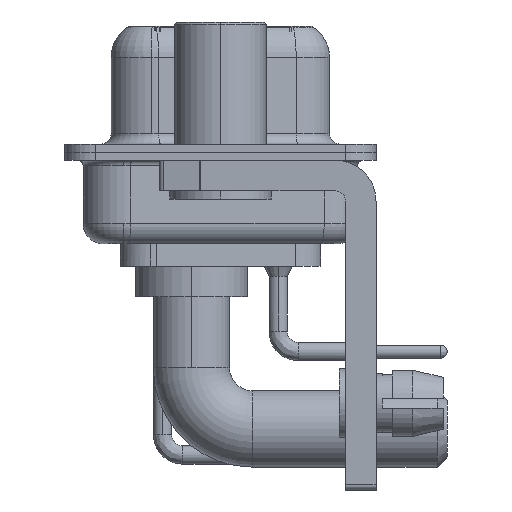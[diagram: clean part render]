
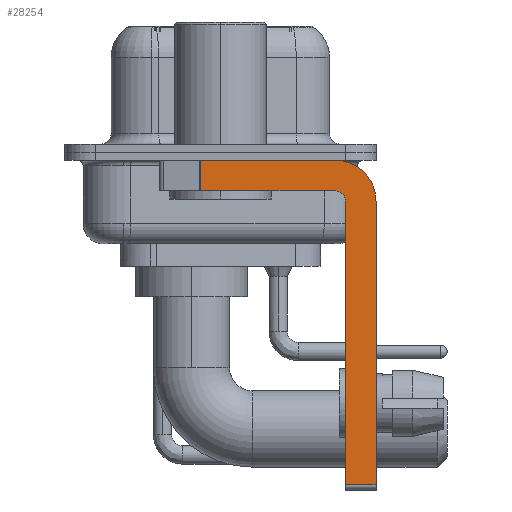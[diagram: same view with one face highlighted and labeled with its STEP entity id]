
A CAD part, left-side view. The second image highlights one B-rep face of the part: STEP entity #28254.
In plain terms, the highlighted planar face has unit normal (-1, 0, 0).
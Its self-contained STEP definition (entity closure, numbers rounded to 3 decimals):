
#24 = CARTESIAN_POINT ( 'NONE',  ( -2.9, -7.65, -2.4 ) ) ;
#41 = VERTEX_POINT ( 'NONE', #19818 ) ;
#48 = EDGE_CURVE ( 'NONE', #21300, #15903, #20177, .T. ) ;
#217 = CARTESIAN_POINT ( 'NONE',  ( -2.9, -5.65, -16.35 ) ) ;
#227 = EDGE_CURVE ( 'NONE', #41, #6944, #7013, .T. ) ;
#390 = CARTESIAN_POINT ( 'NONE',  ( -2.9, -6.15, -16.35 ) ) ;
#1118 = EDGE_CURVE ( 'NONE', #6944, #13479, #3694, .T. ) ;
#1519 = CARTESIAN_POINT ( 'NONE',  ( -2.9, 3., -0.4 ) ) ;
#1580 = ORIENTED_EDGE ( 'NONE', *, *, #1118, .F. ) ;
#2165 = CARTESIAN_POINT ( 'NONE',  ( -2.9, -5.65, -2.4 ) ) ;
#2427 = CARTESIAN_POINT ( 'NONE',  ( -2.9, 0.978, -1.9 ) ) ;
#3694 = CIRCLE ( 'NONE', #24079, 2. ) ;
#4202 = CARTESIAN_POINT ( 'NONE',  ( -2.9, -7.65, -16.35 ) ) ;
#5958 = LINE ( 'NONE', #10878, #18005 ) ;
#6080 = DIRECTION ( 'NONE',  ( 0., -1., 0. ) ) ;
#6709 = EDGE_CURVE ( 'NONE', #13578, #22641, #17053, .T. ) ;
#6944 = VERTEX_POINT ( 'NONE', #26515 ) ;
#6949 = ORIENTED_EDGE ( 'NONE', *, *, #6709, .F. ) ;
#7013 = LINE ( 'NONE', #1519, #30389 ) ;
#8018 = ORIENTED_EDGE ( 'NONE', *, *, #48, .F. ) ;
#10478 = LINE ( 'NONE', #2427, #21187 ) ;
#10837 = DIRECTION ( 'NONE',  ( 0., 0., -1. ) ) ;
#10878 = CARTESIAN_POINT ( 'NONE',  ( -2.9, -7.65, -2.4 ) ) ;
#13140 = ORIENTED_EDGE ( 'NONE', *, *, #227, .F. ) ;
#13209 = DIRECTION ( 'NONE',  ( 1., 0., 0. ) ) ;
#13479 = VERTEX_POINT ( 'NONE', #24 ) ;
#13578 = VERTEX_POINT ( 'NONE', #390 ) ;
#14515 = CARTESIAN_POINT ( 'NONE',  ( -2.9, 0.978, -1.9 ) ) ;
#14539 = CARTESIAN_POINT ( 'NONE',  ( -2.9, -5.65, -1.9 ) ) ;
#14804 = EDGE_LOOP ( 'NONE', ( #13140, #34853, #8018, #33258, #6949, #23740, #29855, #1580 ) ) ;
#15903 = VERTEX_POINT ( 'NONE', #14515 ) ;
#16212 = DIRECTION ( 'NONE',  ( 1., 0., 0. ) ) ;
#17053 = LINE ( 'NONE', #22169, #34877 ) ;
#17980 = CIRCLE ( 'NONE', #29614, 0.5 ) ;
#18005 = VECTOR ( 'NONE', #22196, 1000. ) ;
#19558 = EDGE_CURVE ( 'NONE', #22641, #21300, #17980, .T. ) ;
#19818 = CARTESIAN_POINT ( 'NONE',  ( -2.9, 0.978, -0.4 ) ) ;
#19972 = EDGE_CURVE ( 'NONE', #13479, #21497, #5958, .T. ) ;
#20177 = LINE ( 'NONE', #28390, #25109 ) ;
#21070 = DIRECTION ( 'NONE',  ( 0., -1., 0. ) ) ;
#21187 = VECTOR ( 'NONE', #10837, 1000. ) ;
#21300 = VERTEX_POINT ( 'NONE', #14539 ) ;
#21497 = VERTEX_POINT ( 'NONE', #4202 ) ;
#22169 = CARTESIAN_POINT ( 'NONE',  ( -2.9, -6.15, -16.6 ) ) ;
#22196 = DIRECTION ( 'NONE',  ( 0., 0., -1. ) ) ;
#22641 = VERTEX_POINT ( 'NONE', #33586 ) ;
#22812 = VECTOR ( 'NONE', #6080, 1000. ) ;
#23317 = DIRECTION ( 'NONE',  ( -1., 0., 0. ) ) ;
#23506 = EDGE_CURVE ( 'NONE', #13578, #21497, #30887, .T. ) ;
#23740 = ORIENTED_EDGE ( 'NONE', *, *, #23506, .T. ) ;
#24079 = AXIS2_PLACEMENT_3D ( 'NONE', #2165, #16212, #27338 ) ;
#25109 = VECTOR ( 'NONE', #31300, 1000. ) ;
#25572 = EDGE_CURVE ( 'NONE', #41, #15903, #10478, .T. ) ;
#26515 = CARTESIAN_POINT ( 'NONE',  ( -2.9, -5.65, -0.4 ) ) ;
#27061 = CARTESIAN_POINT ( 'NONE',  ( -2.9, -5.65, -2.4 ) ) ;
#27338 = DIRECTION ( 'NONE',  ( 0., 0., -1. ) ) ;
#27787 = FACE_OUTER_BOUND ( 'NONE', #14804, .T. ) ;
#28254 = ADVANCED_FACE ( 'NONE', ( #27787 ), #31192, .F. ) ;
#28390 = CARTESIAN_POINT ( 'NONE',  ( -2.9, -5.65, -1.9 ) ) ;
#29132 = CARTESIAN_POINT ( 'NONE',  ( -2.9, -5.65, -2.4 ) ) ;
#29614 = AXIS2_PLACEMENT_3D ( 'NONE', #29132, #23317, #31346 ) ;
#29855 = ORIENTED_EDGE ( 'NONE', *, *, #19972, .F. ) ;
#30389 = VECTOR ( 'NONE', #21070, 1000. ) ;
#30887 = LINE ( 'NONE', #217, #22812 ) ;
#31192 = PLANE ( 'NONE',  #31544 ) ;
#31300 = DIRECTION ( 'NONE',  ( 0., 1., 0. ) ) ;
#31346 = DIRECTION ( 'NONE',  ( 0., 0., 1. ) ) ;
#31544 = AXIS2_PLACEMENT_3D ( 'NONE', #27061, #13209, #35447 ) ;
#33258 = ORIENTED_EDGE ( 'NONE', *, *, #19558, .F. ) ;
#33287 = DIRECTION ( 'NONE',  ( 0., 0., 1. ) ) ;
#33586 = CARTESIAN_POINT ( 'NONE',  ( -2.9, -6.15, -2.4 ) ) ;
#34853 = ORIENTED_EDGE ( 'NONE', *, *, #25572, .T. ) ;
#34877 = VECTOR ( 'NONE', #33287, 1000. ) ;
#35447 = DIRECTION ( 'NONE',  ( 0., 0., -1. ) ) ;
